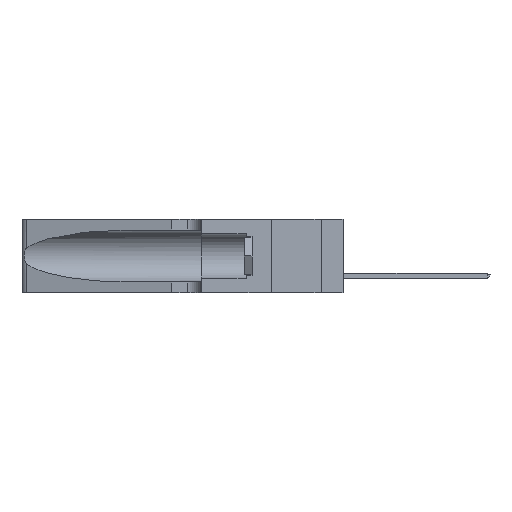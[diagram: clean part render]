
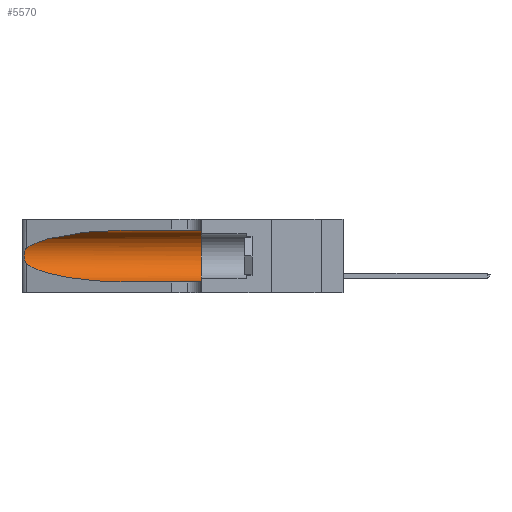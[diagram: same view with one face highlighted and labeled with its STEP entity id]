
A CAD part, left-side view. The second image highlights one B-rep face of the part: STEP entity #5570.
In plain terms, the highlighted cylindrical face has radius 3.308 mm (diameter 6.617 mm), a partial arc.
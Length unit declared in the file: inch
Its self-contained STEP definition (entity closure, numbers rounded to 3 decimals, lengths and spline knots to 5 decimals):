
#1838 = VERTEX_POINT ( 'NONE', #19132 ) ;
#1915 = CARTESIAN_POINT ( 'NONE',  ( 0.25487, 1.22718, 0.22369 ) ) ;
#1918 = AXIS2_PLACEMENT_3D ( 'NONE', #35872, #33146, #20222 ) ;
#2175 = CARTESIAN_POINT ( 'NONE',  ( 0.25487, 1.22718, 0.14631 ) ) ;
#2620 = CARTESIAN_POINT ( 'NONE',  ( 0.25787, 1.23484, 0.2124 ) ) ;
#2684 = CYLINDRICAL_SURFACE ( 'NONE', #44444, 0.13025 ) ;
#3582 = DIRECTION ( 'NONE',  ( 0., -1., 0. ) ) ;
#5159 = CARTESIAN_POINT ( 'NONE',  ( 0.26075, 1.23896, 0.19203 ) ) ;
#5214 = ORIENTED_EDGE ( 'NONE', *, *, #25814, .T. ) ;
#5570 = ADVANCED_FACE ( 'NONE', ( #19923 ), #2684, .F. ) ;
#5978 = CARTESIAN_POINT ( 'NONE',  ( 0.18966, 0.96281, 0.31525 ) ) ;
#7132 = ORIENTED_EDGE ( 'NONE', *, *, #23790, .T. ) ;
#7609 = ORIENTED_EDGE ( 'NONE', *, *, #28581, .F. ) ;
#8048 = VERTEX_POINT ( 'NONE', #1915 ) ;
#9495 = CARTESIAN_POINT ( 'NONE',  ( 0.25555, 1.22994, 0.2215 ) ) ;
#9842 = VERTEX_POINT ( 'NONE', #41875 ) ;
#9875 = CARTESIAN_POINT ( 'NONE',  ( 0.1305, 0.72297, 0.31525 ) ) ;
#11431 = VERTEX_POINT ( 'NONE', #25343 ) ;
#13076 = CARTESIAN_POINT ( 'NONE',  ( 0.1305, 1.61858, 0.31525 ) ) ;
#15327 = EDGE_LOOP ( 'NONE', ( #7132, #32162, #41546, #5214, #7609, #23959 ) ) ;
#16670 = CARTESIAN_POINT ( 'NONE',  ( 0.2373, 1.15595, 0.08982 ) ) ;
#16809 = CARTESIAN_POINT ( 'NONE',  ( 0.25639, 1.23184, 0.21858 ) ) ;
#17225 =( BOUNDED_CURVE ( )  B_SPLINE_CURVE ( 3, ( #23925, #16670, #42156, #20257 ),
 .UNSPECIFIED., .F., .F. ) 
 B_SPLINE_CURVE_WITH_KNOTS ( ( 4, 4 ),
 ( 3.44316, 4.71239 ),
 .UNSPECIFIED. ) 
 CURVE ( )  GEOMETRIC_REPRESENTATION_ITEM ( )  RATIONAL_B_SPLINE_CURVE ( ( 1., 0.87, 0.87, 1. ) ) 
 REPRESENTATION_ITEM ( '' )  );
#18106 = DIRECTION ( 'NONE',  ( 0., -1., 0. ) ) ;
#19132 = CARTESIAN_POINT ( 'NONE',  ( 0.1305, 0.72297, 0.31525 ) ) ;
#19923 = FACE_OUTER_BOUND ( 'NONE', #15327, .T. ) ;
#20072 = CARTESIAN_POINT ( 'NONE',  ( 0.25487, 1.22718, 0.14631 ) ) ;
#20222 = DIRECTION ( 'NONE',  ( 0., 0., 1. ) ) ;
#20257 = CARTESIAN_POINT ( 'NONE',  ( 0.1305, 0.72297, 0.05475 ) ) ;
#20536 = CARTESIAN_POINT ( 'NONE',  ( 0.25854, 1.2359, 0.20912 ) ) ;
#21151 = CIRCLE ( 'NONE', #1918, 0.13025 ) ;
#21241 = CARTESIAN_POINT ( 'NONE',  ( 0.25856, 1.23593, 0.16098 ) ) ;
#21415 = LINE ( 'NONE', #41601, #42057 ) ;
#21476 = CARTESIAN_POINT ( 'NONE',  ( 0.25555, 1.22993, 0.14849 ) ) ;
#21947 = B_SPLINE_CURVE_WITH_KNOTS ( 'NONE', 3,
 ( #37666, #9495, #16809, #2620, #20536, #35023, #5159, #23006, #38953, #21241, #24506, #31441, #21476, #2175 ),
 .UNSPECIFIED., .F., .F.,
 ( 4, 2, 2, 2, 2, 2, 4 ),
 ( 0., 0.00027, 0.00053, 0.00107, 0.0016, 0.00187, 0.00214 ),
 .UNSPECIFIED. ) ;
#23006 = CARTESIAN_POINT ( 'NONE',  ( 0.26075, 1.23896, 0.178 ) ) ;
#23666 = CARTESIAN_POINT ( 'NONE',  ( 0.25487, 1.22718, 0.22369 ) ) ;
#23790 = EDGE_CURVE ( 'NONE', #1838, #8048, #45444, .T. ) ;
#23925 = CARTESIAN_POINT ( 'NONE',  ( 0.25487, 1.22718, 0.14631 ) ) ;
#23959 = ORIENTED_EDGE ( 'NONE', *, *, #42959, .F. ) ;
#24506 = CARTESIAN_POINT ( 'NONE',  ( 0.25789, 1.23486, 0.15765 ) ) ;
#25343 = CARTESIAN_POINT ( 'NONE',  ( 0.1305, 0.35, 0.31525 ) ) ;
#25814 = EDGE_CURVE ( 'NONE', #38924, #9842, #21415, .T. ) ;
#26537 = EDGE_CURVE ( 'NONE', #45907, #38924, #17225, .T. ) ;
#27815 = VECTOR ( 'NONE', #18106, 39.37008 ) ;
#28581 = EDGE_CURVE ( 'NONE', #11431, #9842, #21151, .T. ) ;
#28748 = DIRECTION ( 'NONE',  ( 0., -1., 0. ) ) ;
#30865 = CARTESIAN_POINT ( 'NONE',  ( 0.2373, 1.15595, 0.28018 ) ) ;
#31441 = CARTESIAN_POINT ( 'NONE',  ( 0.25639, 1.23186, 0.15144 ) ) ;
#32141 = EDGE_CURVE ( 'NONE', #8048, #45907, #21947, .T. ) ;
#32162 = ORIENTED_EDGE ( 'NONE', *, *, #32141, .T. ) ;
#33146 = DIRECTION ( 'NONE',  ( 0., 1., 0. ) ) ;
#35023 = CARTESIAN_POINT ( 'NONE',  ( 0.26018, 1.23835, 0.19895 ) ) ;
#35872 = CARTESIAN_POINT ( 'NONE',  ( 0.1305, 0.35, 0.185 ) ) ;
#37666 = CARTESIAN_POINT ( 'NONE',  ( 0.25487, 1.22718, 0.22369 ) ) ;
#38425 = LINE ( 'NONE', #13076, #27815 ) ;
#38924 = VERTEX_POINT ( 'NONE', #43701 ) ;
#38953 = CARTESIAN_POINT ( 'NONE',  ( 0.26017, 1.23833, 0.17102 ) ) ;
#39087 = CARTESIAN_POINT ( 'NONE',  ( 0.1305, 1.61858, 0.185 ) ) ;
#41546 = ORIENTED_EDGE ( 'NONE', *, *, #26537, .T. ) ;
#41601 = CARTESIAN_POINT ( 'NONE',  ( 0.1305, 1.61858, 0.05475 ) ) ;
#41875 = CARTESIAN_POINT ( 'NONE',  ( 0.1305, 0.35, 0.05475 ) ) ;
#42057 = VECTOR ( 'NONE', #28748, 39.37008 ) ;
#42156 = CARTESIAN_POINT ( 'NONE',  ( 0.18966, 0.96281, 0.05475 ) ) ;
#42959 = EDGE_CURVE ( 'NONE', #1838, #11431, #38425, .T. ) ;
#43701 = CARTESIAN_POINT ( 'NONE',  ( 0.1305, 0.72297, 0.05475 ) ) ;
#44444 = AXIS2_PLACEMENT_3D ( 'NONE', #39087, #3582, #45617 ) ;
#45444 =( BOUNDED_CURVE ( )  B_SPLINE_CURVE ( 3, ( #9875, #5978, #30865, #23666 ),
 .UNSPECIFIED., .F., .F. ) 
 B_SPLINE_CURVE_WITH_KNOTS ( ( 4, 4 ),
 ( 1.5708, 2.84003 ),
 .UNSPECIFIED. ) 
 CURVE ( )  GEOMETRIC_REPRESENTATION_ITEM ( )  RATIONAL_B_SPLINE_CURVE ( ( 1., 0.87, 0.87, 1. ) ) 
 REPRESENTATION_ITEM ( '' )  );
#45617 = DIRECTION ( 'NONE',  ( 0., 0., -1. ) ) ;
#45907 = VERTEX_POINT ( 'NONE', #20072 ) ;
